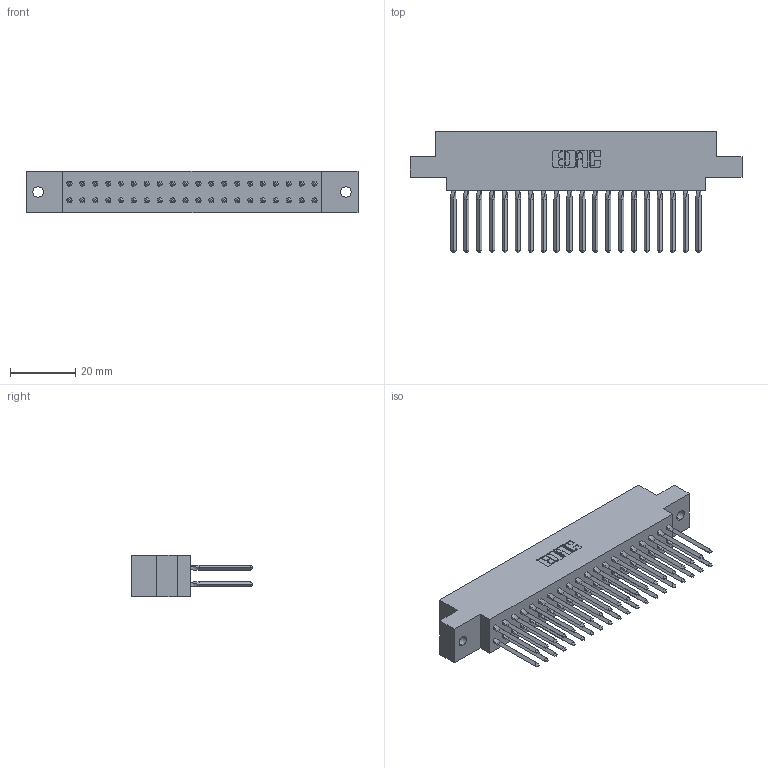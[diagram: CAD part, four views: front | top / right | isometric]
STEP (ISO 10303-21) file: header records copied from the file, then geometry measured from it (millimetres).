
FILE_DESCRIPTION (( 'STEP AP203' ), '1' );
FILE_NAME ('317-040-542-802.STEP', '2020-02-28T00:33:20', ( '' ), ( '' ), 'SwSTEP 2.0', 'SolidWorks 2016', '' );
FILE_SCHEMA (( 'CONFIG_CONTROL_DESIGN' ));
Length unit declared in the file: inch
Products named in the file (3): 317-040-542-802; 317-290-003_542; 317 Part_.144 Dia
Assembly tree (41 placements, depth 2):
  317-040-542-802
    317 Part_.144 Dia
    317-290-003_542  x40
Bounding box: 101.96 x 37.34 x 12.7 mm (x, y, z)
Volume: 15962.9 mm3; surface area: 21225.7 mm2
Topology: 41 solids, 41 shells, 2382 faces, 6675 edges, 4262 vertices
Faces by surface type: plane 1898, cylinder 324, bspline 160
Entity records: 30999 total; most frequent: CARTESIAN_POINT 5653, ORIENTED_EDGE 5316, DIRECTION 4510, EDGE_CURVE 2658, LINE 2488, VECTOR 2488, VERTEX_POINT 1766, AXIS2_PLACEMENT_3D 1011
